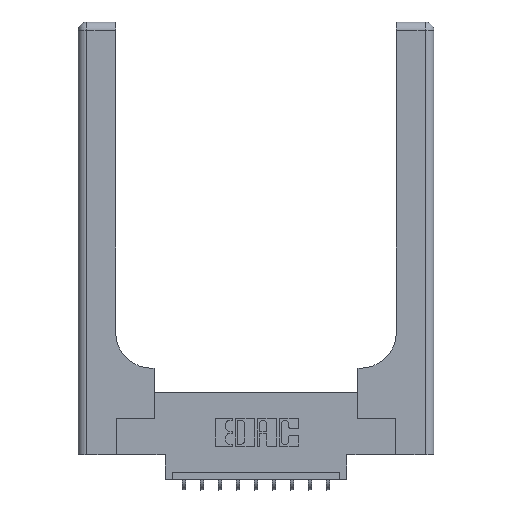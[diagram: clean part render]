
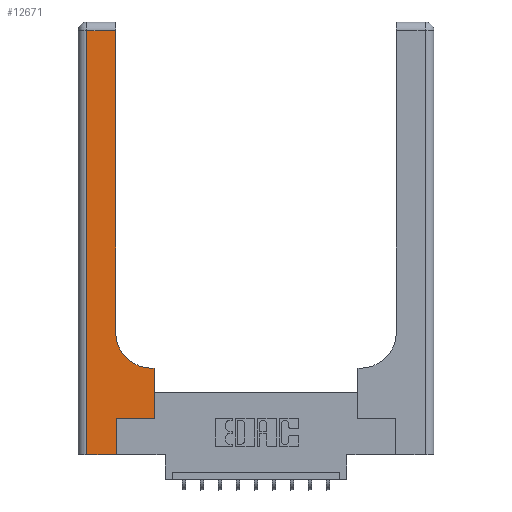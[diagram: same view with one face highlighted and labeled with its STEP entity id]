
A CAD part, top view. The second image highlights one B-rep face of the part: STEP entity #12671.
In plain terms, the highlighted planar face has unit normal (0, 0, 1).
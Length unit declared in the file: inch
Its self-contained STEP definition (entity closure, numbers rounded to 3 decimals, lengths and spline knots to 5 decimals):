
#292 = VERTEX_POINT ( 'NONE', #11376 ) ;
#365 = DIRECTION ( 'NONE',  ( -1., 0., 0. ) ) ;
#1076 = DIRECTION ( 'NONE',  ( 0., 1., 0. ) ) ;
#1092 = DIRECTION ( 'NONE',  ( 1., 0., 0. ) ) ;
#1120 = EDGE_CURVE ( 'NONE', #14444, #1535, #9720, .T. ) ;
#1170 = VERTEX_POINT ( 'NONE', #1672 ) ;
#1373 = FACE_OUTER_BOUND ( 'NONE', #15146, .T. ) ;
#1535 = VERTEX_POINT ( 'NONE', #10941 ) ;
#1548 = AXIS2_PLACEMENT_3D ( 'NONE', #9509, #2362, #10708 ) ;
#1616 = VECTOR ( 'NONE', #9010, 39.37008 ) ;
#1672 = CARTESIAN_POINT ( 'NONE',  ( 0.51, 0.6, 0.37 ) ) ;
#1875 = LINE ( 'NONE', #6488, #11006 ) ;
#2350 = LINE ( 'NONE', #10079, #8377 ) ;
#2362 = DIRECTION ( 'NONE',  ( 0., 0., -1. ) ) ;
#2622 = EDGE_CURVE ( 'NONE', #1535, #3087, #14869, .T. ) ;
#2895 = ORIENTED_EDGE ( 'NONE', *, *, #5993, .T. ) ;
#2958 = VERTEX_POINT ( 'NONE', #13741 ) ;
#3051 = VERTEX_POINT ( 'NONE', #13890 ) ;
#3087 = VERTEX_POINT ( 'NONE', #9223 ) ;
#3673 = VECTOR ( 'NONE', #1076, 39.37008 ) ;
#3861 = EDGE_CURVE ( 'NONE', #292, #9326, #2350, .T. ) ;
#3905 = EDGE_CURVE ( 'NONE', #3051, #2958, #4835, .T. ) ;
#3906 = VECTOR ( 'NONE', #14273, 39.37008 ) ;
#3993 = DIRECTION ( 'NONE',  ( 0., -1., 0. ) ) ;
#4835 = LINE ( 'NONE', #14901, #1616 ) ;
#5462 = CARTESIAN_POINT ( 'NONE',  ( 0., 3., 0.37 ) ) ;
#5993 = EDGE_CURVE ( 'NONE', #2958, #14444, #8166, .T. ) ;
#6168 = ORIENTED_EDGE ( 'NONE', *, *, #2622, .T. ) ;
#6391 = CARTESIAN_POINT ( 'NONE',  ( 0., 2.94, 0.37 ) ) ;
#6488 = CARTESIAN_POINT ( 'NONE',  ( 0.265, 0., 0.37 ) ) ;
#7229 = CARTESIAN_POINT ( 'NONE',  ( 0.26, 0.6, 0.37 ) ) ;
#7489 = LINE ( 'NONE', #7229, #3906 ) ;
#7777 = ORIENTED_EDGE ( 'NONE', *, *, #10225, .T. ) ;
#7811 = VECTOR ( 'NONE', #365, 39.37008 ) ;
#7898 = DIRECTION ( 'NONE',  ( -1., 0., 0. ) ) ;
#8166 = LINE ( 'NONE', #6391, #7811 ) ;
#8296 = CARTESIAN_POINT ( 'NONE',  ( 0., 0., 0.37 ) ) ;
#8377 = VECTOR ( 'NONE', #12414, 39.37008 ) ;
#9010 = DIRECTION ( 'NONE',  ( 0., 1., 0. ) ) ;
#9223 = CARTESIAN_POINT ( 'NONE',  ( 0.265, 0., 0.37 ) ) ;
#9326 = VERTEX_POINT ( 'NONE', #13895 ) ;
#9509 = CARTESIAN_POINT ( 'NONE',  ( 0.51, 0.85, 0.37 ) ) ;
#9720 = LINE ( 'NONE', #12297, #12510 ) ;
#9958 = DIRECTION ( 'NONE',  ( 0., 1., 0. ) ) ;
#10079 = CARTESIAN_POINT ( 'NONE',  ( 0.265, 0.25, 0.37 ) ) ;
#10225 = EDGE_CURVE ( 'NONE', #1170, #3051, #13744, .T. ) ;
#10248 = EDGE_CURVE ( 'NONE', #10574, #1170, #7489, .T. ) ;
#10574 = VERTEX_POINT ( 'NONE', #11465 ) ;
#10656 = ORIENTED_EDGE ( 'NONE', *, *, #1120, .T. ) ;
#10708 = DIRECTION ( 'NONE',  ( 1., 0., 0. ) ) ;
#10941 = CARTESIAN_POINT ( 'NONE',  ( 0.06, 0., 0.37 ) ) ;
#11006 = VECTOR ( 'NONE', #9958, 39.37008 ) ;
#11341 = VECTOR ( 'NONE', #1092, 39.37008 ) ;
#11376 = CARTESIAN_POINT ( 'NONE',  ( 0.265, 0.25, 0.37 ) ) ;
#11437 = EDGE_CURVE ( 'NONE', #9326, #10574, #13141, .T. ) ;
#11465 = CARTESIAN_POINT ( 'NONE',  ( 0.528, 0.6, 0.37 ) ) ;
#11600 = ORIENTED_EDGE ( 'NONE', *, *, #3861, .T. ) ;
#11749 = ORIENTED_EDGE ( 'NONE', *, *, #10248, .T. ) ;
#12242 = AXIS2_PLACEMENT_3D ( 'NONE', #5462, #14950, #7898 ) ;
#12297 = CARTESIAN_POINT ( 'NONE',  ( 0.06, 3., 0.37 ) ) ;
#12335 = ORIENTED_EDGE ( 'NONE', *, *, #15281, .T. ) ;
#12414 = DIRECTION ( 'NONE',  ( 1., 0., 0. ) ) ;
#12510 = VECTOR ( 'NONE', #3993, 39.37008 ) ;
#12564 = PLANE ( 'NONE',  #12242 ) ;
#12671 = ADVANCED_FACE ( 'NONE', ( #1373 ), #12564, .F. ) ;
#13141 = LINE ( 'NONE', #14142, #3673 ) ;
#13741 = CARTESIAN_POINT ( 'NONE',  ( 0.26, 2.94, 0.37 ) ) ;
#13744 = CIRCLE ( 'NONE', #1548, 0.25 ) ;
#13890 = CARTESIAN_POINT ( 'NONE',  ( 0.26, 0.85, 0.37 ) ) ;
#13895 = CARTESIAN_POINT ( 'NONE',  ( 0.528, 0.25, 0.37 ) ) ;
#14142 = CARTESIAN_POINT ( 'NONE',  ( 0.528, 0.25, 0.37 ) ) ;
#14273 = DIRECTION ( 'NONE',  ( -1., 0., 0. ) ) ;
#14444 = VERTEX_POINT ( 'NONE', #15422 ) ;
#14869 = LINE ( 'NONE', #8296, #11341 ) ;
#14901 = CARTESIAN_POINT ( 'NONE',  ( 0.26, 3., 0.37 ) ) ;
#14950 = DIRECTION ( 'NONE',  ( 0., 0., -1. ) ) ;
#15029 = ORIENTED_EDGE ( 'NONE', *, *, #3905, .T. ) ;
#15146 = EDGE_LOOP ( 'NONE', ( #15029, #2895, #10656, #6168, #12335, #11600, #15433, #11749, #7777 ) ) ;
#15281 = EDGE_CURVE ( 'NONE', #3087, #292, #1875, .T. ) ;
#15422 = CARTESIAN_POINT ( 'NONE',  ( 0.06, 2.94, 0.37 ) ) ;
#15433 = ORIENTED_EDGE ( 'NONE', *, *, #11437, .T. ) ;
